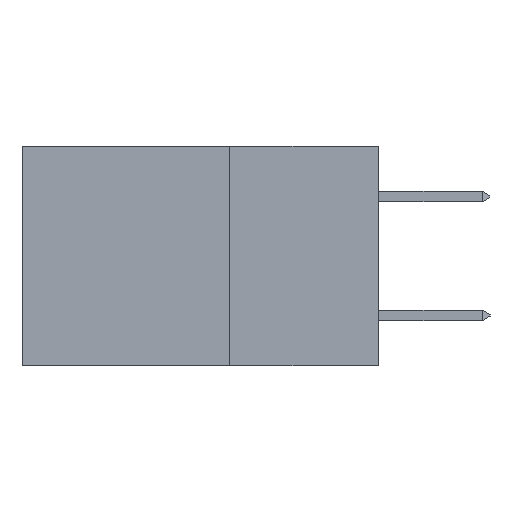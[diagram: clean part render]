
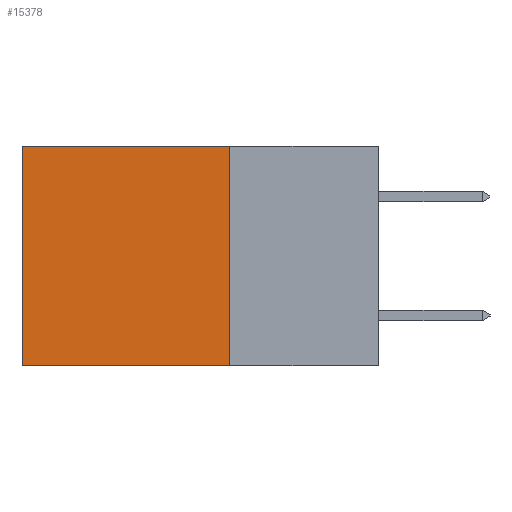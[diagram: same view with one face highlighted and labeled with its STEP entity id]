
A CAD part, left-side view. The second image highlights one B-rep face of the part: STEP entity #15378.
In plain terms, the highlighted planar face has unit normal (-1, 0, 0).
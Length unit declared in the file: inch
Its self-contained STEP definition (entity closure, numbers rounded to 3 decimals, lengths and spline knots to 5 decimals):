
#606 = AXIS2_PLACEMENT_3D ( 'NONE', #15984, #10104, #883 ) ;
#883 = DIRECTION ( 'NONE',  ( 0., 0., -1. ) ) ;
#1224 = LINE ( 'NONE', #4307, #16355 ) ;
#1435 = VERTEX_POINT ( 'NONE', #2604 ) ;
#2604 = CARTESIAN_POINT ( 'NONE',  ( 0.2615, 0.6, -0.37 ) ) ;
#3473 = FACE_OUTER_BOUND ( 'NONE', #19187, .T. ) ;
#4307 = CARTESIAN_POINT ( 'NONE',  ( 0.2615, 0.25, -0.37 ) ) ;
#6187 = VECTOR ( 'NONE', #13726, 39.37008 ) ;
#6607 = EDGE_CURVE ( 'NONE', #15772, #9168, #18982, .T. ) ;
#9097 = ORIENTED_EDGE ( 'NONE', *, *, #15054, .T. ) ;
#9168 = VERTEX_POINT ( 'NONE', #19280 ) ;
#9505 = CARTESIAN_POINT ( 'NONE',  ( 0.2615, 0.25, -0.37 ) ) ;
#9656 = VECTOR ( 'NONE', #11071, 39.37008 ) ;
#10104 = DIRECTION ( 'NONE',  ( 1., 0., 0. ) ) ;
#10115 = LINE ( 'NONE', #18488, #9656 ) ;
#10938 = LINE ( 'NONE', #9505, #18370 ) ;
#10985 = EDGE_CURVE ( 'NONE', #15772, #15519, #10938, .T. ) ;
#11071 = DIRECTION ( 'NONE',  ( 0., 0., -1. ) ) ;
#12093 = ORIENTED_EDGE ( 'NONE', *, *, #6607, .T. ) ;
#12488 = DIRECTION ( 'NONE',  ( 0., 0., -1. ) ) ;
#13726 = DIRECTION ( 'NONE',  ( 0., 1., 0. ) ) ;
#13793 = CARTESIAN_POINT ( 'NONE',  ( 0.2615, 0.25, 0. ) ) ;
#14161 = CARTESIAN_POINT ( 'NONE',  ( 0.2615, 0.25, 0. ) ) ;
#14665 = EDGE_CURVE ( 'NONE', #15519, #1435, #1224, .T. ) ;
#14734 = DIRECTION ( 'NONE',  ( 0., 1., 0. ) ) ;
#14828 = CARTESIAN_POINT ( 'NONE',  ( 0.2615, 0.25, -0.37 ) ) ;
#15054 = EDGE_CURVE ( 'NONE', #9168, #1435, #10115, .T. ) ;
#15112 = ORIENTED_EDGE ( 'NONE', *, *, #10985, .F. ) ;
#15378 = ADVANCED_FACE ( 'NONE', ( #3473 ), #19002, .F. ) ;
#15519 = VERTEX_POINT ( 'NONE', #14828 ) ;
#15772 = VERTEX_POINT ( 'NONE', #14161 ) ;
#15984 = CARTESIAN_POINT ( 'NONE',  ( 0.2615, 0.25, -0.37 ) ) ;
#16355 = VECTOR ( 'NONE', #14734, 39.37008 ) ;
#18370 = VECTOR ( 'NONE', #12488, 39.37008 ) ;
#18488 = CARTESIAN_POINT ( 'NONE',  ( 0.2615, 0.6, -0.37 ) ) ;
#18830 = ORIENTED_EDGE ( 'NONE', *, *, #14665, .F. ) ;
#18982 = LINE ( 'NONE', #13793, #6187 ) ;
#19002 = PLANE ( 'NONE',  #606 ) ;
#19187 = EDGE_LOOP ( 'NONE', ( #9097, #18830, #15112, #12093 ) ) ;
#19280 = CARTESIAN_POINT ( 'NONE',  ( 0.2615, 0.6, 0. ) ) ;
